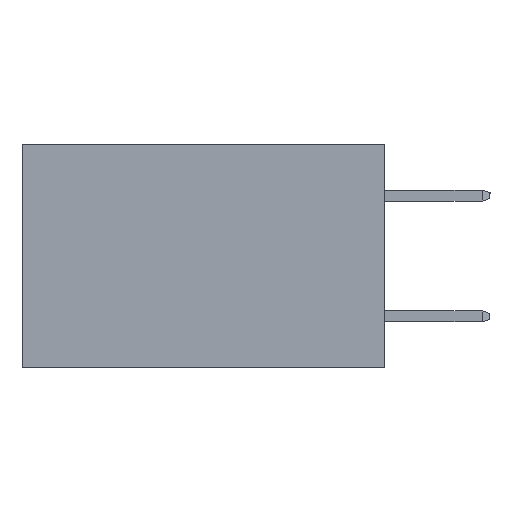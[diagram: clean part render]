
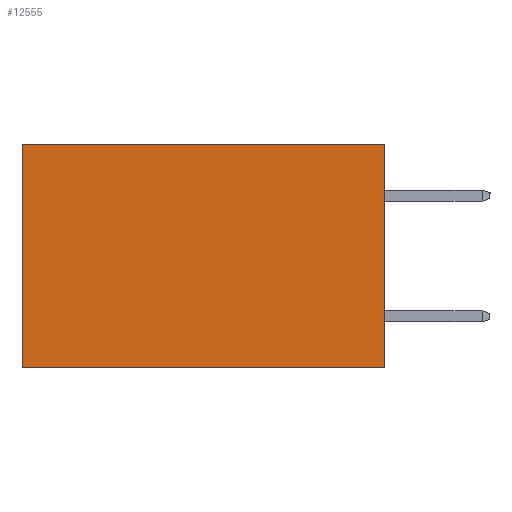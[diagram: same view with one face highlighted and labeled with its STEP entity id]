
A CAD part, left-side view. The second image highlights one B-rep face of the part: STEP entity #12555.
In plain terms, the highlighted planar face has unit normal (-1, 0, 0).
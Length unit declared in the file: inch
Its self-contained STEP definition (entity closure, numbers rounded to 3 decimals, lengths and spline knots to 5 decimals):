
#162 = LINE ( 'NONE', #1578, #13601 ) ;
#633 = CARTESIAN_POINT ( 'NONE',  ( 0.2615, 0., -0.37 ) ) ;
#1254 = CARTESIAN_POINT ( 'NONE',  ( 0.2615, 0., 0. ) ) ;
#1578 = CARTESIAN_POINT ( 'NONE',  ( 0.2615, 0.6, -0.37 ) ) ;
#1862 = LINE ( 'NONE', #8451, #12618 ) ;
#2562 = ORIENTED_EDGE ( 'NONE', *, *, #7904, .T. ) ;
#3240 = CARTESIAN_POINT ( 'NONE',  ( 0.2615, 0.6, -0.37 ) ) ;
#3472 = ORIENTED_EDGE ( 'NONE', *, *, #10115, .F. ) ;
#3938 = PLANE ( 'NONE',  #8059 ) ;
#4014 = VERTEX_POINT ( 'NONE', #10943 ) ;
#4415 = CARTESIAN_POINT ( 'NONE',  ( 0.2615, 0., -0.37 ) ) ;
#4671 = DIRECTION ( 'NONE',  ( 0., 0., -1. ) ) ;
#6605 = FACE_OUTER_BOUND ( 'NONE', #16386, .T. ) ;
#7904 = EDGE_CURVE ( 'NONE', #4014, #14866, #162, .T. ) ;
#8059 = AXIS2_PLACEMENT_3D ( 'NONE', #16135, #12136, #9369 ) ;
#8451 = CARTESIAN_POINT ( 'NONE',  ( 0.2615, 0., -0.37 ) ) ;
#8601 = DIRECTION ( 'NONE',  ( 0., 0., -1. ) ) ;
#8975 = VERTEX_POINT ( 'NONE', #17072 ) ;
#9369 = DIRECTION ( 'NONE',  ( 0., 0., -1. ) ) ;
#10115 = EDGE_CURVE ( 'NONE', #12820, #14866, #1862, .T. ) ;
#10943 = CARTESIAN_POINT ( 'NONE',  ( 0.2615, 0.6, 0. ) ) ;
#11196 = LINE ( 'NONE', #4415, #15241 ) ;
#11797 = EDGE_CURVE ( 'NONE', #8975, #4014, #11842, .T. ) ;
#11842 = LINE ( 'NONE', #1254, #17456 ) ;
#12121 = DIRECTION ( 'NONE',  ( 0., 1., 0. ) ) ;
#12136 = DIRECTION ( 'NONE',  ( 1., 0., 0. ) ) ;
#12555 = ADVANCED_FACE ( 'NONE', ( #6605 ), #3938, .F. ) ;
#12618 = VECTOR ( 'NONE', #14061, 39.37008 ) ;
#12820 = VERTEX_POINT ( 'NONE', #633 ) ;
#13565 = ORIENTED_EDGE ( 'NONE', *, *, #13687, .F. ) ;
#13601 = VECTOR ( 'NONE', #8601, 39.37008 ) ;
#13687 = EDGE_CURVE ( 'NONE', #8975, #12820, #11196, .T. ) ;
#14061 = DIRECTION ( 'NONE',  ( 0., 1., 0. ) ) ;
#14592 = ORIENTED_EDGE ( 'NONE', *, *, #11797, .T. ) ;
#14866 = VERTEX_POINT ( 'NONE', #3240 ) ;
#15241 = VECTOR ( 'NONE', #4671, 39.37008 ) ;
#16135 = CARTESIAN_POINT ( 'NONE',  ( 0.2615, 0., -0.37 ) ) ;
#16386 = EDGE_LOOP ( 'NONE', ( #2562, #3472, #13565, #14592 ) ) ;
#17072 = CARTESIAN_POINT ( 'NONE',  ( 0.2615, 0., 0. ) ) ;
#17456 = VECTOR ( 'NONE', #12121, 39.37008 ) ;
